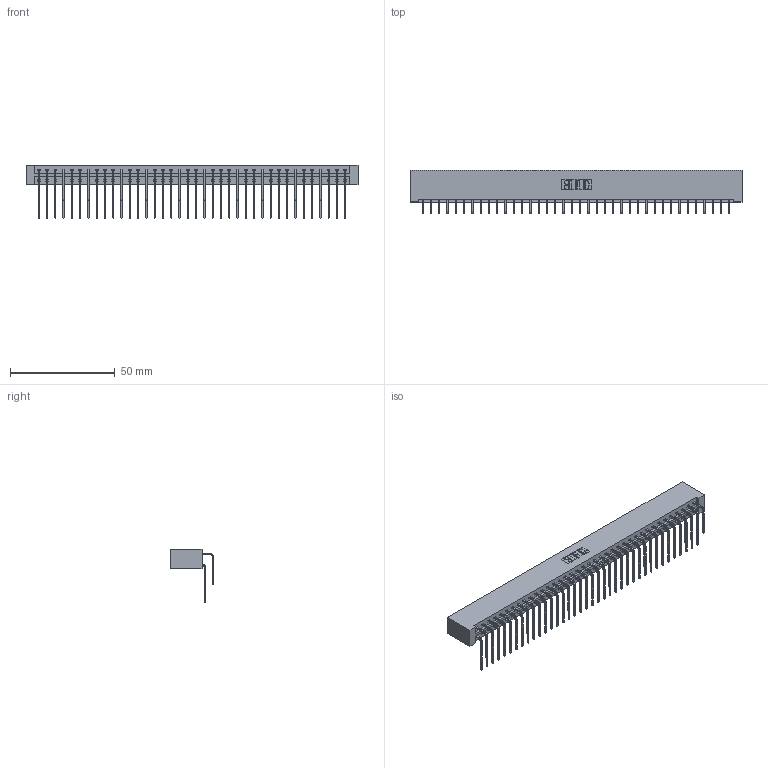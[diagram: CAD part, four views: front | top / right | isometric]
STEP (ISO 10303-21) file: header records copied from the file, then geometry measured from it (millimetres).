
FILE_DESCRIPTION (( 'STEP AP203' ), '1' );
FILE_NAME ('833-076-559-201.STEP', '2020-06-05T19:06:35', ( '' ), ( '' ), 'SwSTEP 2.0', 'SolidWorks 2020', '' );
FILE_SCHEMA (( 'CONFIG_CONTROL_DESIGN' ));
Length unit declared in the file: inch
Products named in the file (4): 345-292-001_558 559 Tail - 1; 833 Part_Lugless; 345-292-001_559 Tail - 2; 833-076-559-201
Assembly tree (77 placements, depth 2):
  833-076-559-201
    833 Part_Lugless
    345-292-001_558 559 Tail - 1  x38
    345-292-001_559 Tail - 2  x38
Bounding box: 158.83 x 20.9 x 25.53 mm (x, y, z)
Volume: 17248.5 mm3; surface area: 22557.2 mm2
Topology: 77 solids, 77 shells, 4210 faces, 12523 edges, 8246 vertices
Faces by surface type: plane 2954, cylinder 1256
Entity records: 26471 total; most frequent: CARTESIAN_POINT 4441, ORIENTED_EDGE 4326, DIRECTION 3775, EDGE_CURVE 2163, LINE 2003, VECTOR 2003, VERTEX_POINT 1438, AXIS2_PLACEMENT_3D 886
